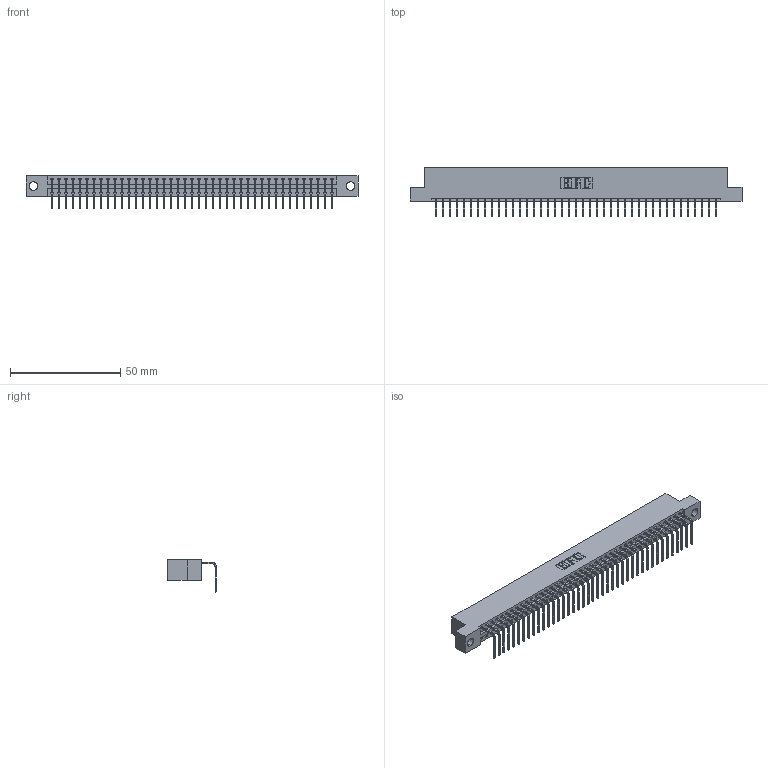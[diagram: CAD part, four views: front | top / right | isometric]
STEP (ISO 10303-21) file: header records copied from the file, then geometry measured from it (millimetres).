
FILE_DESCRIPTION (( 'STEP AP203' ), '1' );
FILE_NAME ('346-041-558-104.STEP', '2018-08-24T12:03:14', ( '' ), ( '' ), 'SwSTEP 2.0', 'SolidWorks 2016', '' );
FILE_SCHEMA (( 'CONFIG_CONTROL_DESIGN' ));
Length unit declared in the file: inch
Products named in the file (3): 346 Part_Flush Mounting Lugs - 0.156 Dia-TH; 345-292-001_558 Tail - 2; 346-041-558-104
Assembly tree (42 placements, depth 2):
  346-041-558-104
    346 Part_Flush Mounting Lugs - 0.156 Dia-TH
    345-292-001_558 Tail - 2  x41
Bounding box: 150.75 x 22.16 x 14.73 mm (x, y, z)
Volume: 14471.9 mm3; surface area: 18697.1 mm2
Topology: 42 solids, 42 shells, 2582 faces, 7791 edges, 5138 vertices
Faces by surface type: plane 1798, cylinder 784
Entity records: 25667 total; most frequent: CARTESIAN_POINT 4407, ORIENTED_EDGE 4382, DIRECTION 3889, EDGE_CURVE 2191, LINE 1895, VECTOR 1895, VERTEX_POINT 1458, AXIS2_PLACEMENT_3D 997
